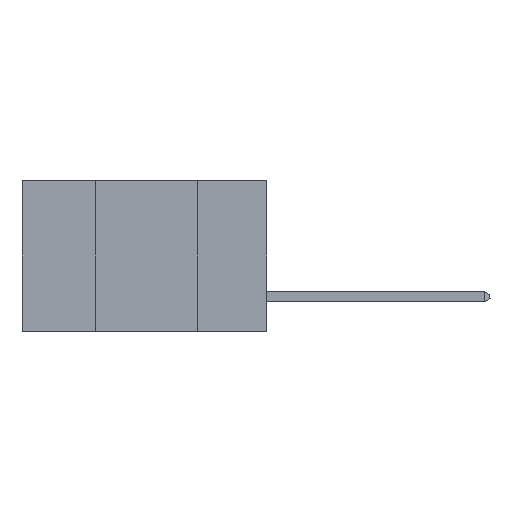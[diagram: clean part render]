
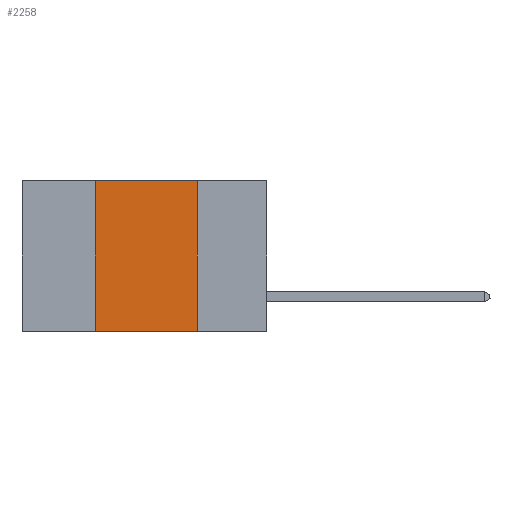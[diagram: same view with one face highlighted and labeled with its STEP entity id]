
A CAD part, left-side view. The second image highlights one B-rep face of the part: STEP entity #2258.
In plain terms, the highlighted planar face has unit normal (-1, 0, 0).
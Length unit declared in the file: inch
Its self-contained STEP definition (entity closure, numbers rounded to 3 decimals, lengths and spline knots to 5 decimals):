
#141 = ORIENTED_EDGE ( 'NONE', *, *, #20938, .F. ) ;
#144 = VERTEX_POINT ( 'NONE', #7579 ) ;
#850 = EDGE_CURVE ( 'NONE', #144, #875, #19099, .T. ) ;
#875 = VERTEX_POINT ( 'NONE', #9905 ) ;
#2085 = VECTOR ( 'NONE', #15991, 39.37008 ) ;
#2258 = ADVANCED_FACE ( 'NONE', ( #5302 ), #19737, .F. ) ;
#3033 = ORIENTED_EDGE ( 'NONE', *, *, #5304, .F. ) ;
#4265 = EDGE_LOOP ( 'NONE', ( #11182, #3033, #141, #21207 ) ) ;
#4386 = DIRECTION ( 'NONE',  ( 0., -1., 0. ) ) ;
#5198 = CARTESIAN_POINT ( 'NONE',  ( 0., 0.42, 0. ) ) ;
#5302 = FACE_OUTER_BOUND ( 'NONE', #4265, .T. ) ;
#5304 = EDGE_CURVE ( 'NONE', #12394, #144, #10483, .T. ) ;
#7237 = VECTOR ( 'NONE', #17826, 39.37008 ) ;
#7579 = CARTESIAN_POINT ( 'NONE',  ( 0., 0.17, 0. ) ) ;
#9636 = VECTOR ( 'NONE', #4386, 39.37008 ) ;
#9807 = DIRECTION ( 'NONE',  ( 1., 0., 0. ) ) ;
#9905 = CARTESIAN_POINT ( 'NONE',  ( 0., 0.17, -0.37 ) ) ;
#10110 = VECTOR ( 'NONE', #11471, 39.37008 ) ;
#10138 = CARTESIAN_POINT ( 'NONE',  ( 0., 0.6, -0.37 ) ) ;
#10392 = CARTESIAN_POINT ( 'NONE',  ( 0., 0.42, -0.37 ) ) ;
#10483 = LINE ( 'NONE', #16244, #2085 ) ;
#11182 = ORIENTED_EDGE ( 'NONE', *, *, #850, .F. ) ;
#11471 = DIRECTION ( 'NONE',  ( 0., 0., 1. ) ) ;
#11735 = CARTESIAN_POINT ( 'NONE',  ( 0., 0.17, 0. ) ) ;
#11829 = DIRECTION ( 'NONE',  ( 0., 0., -1. ) ) ;
#12394 = VERTEX_POINT ( 'NONE', #20597 ) ;
#15991 = DIRECTION ( 'NONE',  ( 0., -1., 0. ) ) ;
#16244 = CARTESIAN_POINT ( 'NONE',  ( 0., 0.6, 0. ) ) ;
#17371 = EDGE_CURVE ( 'NONE', #22527, #875, #18966, .T. ) ;
#17826 = DIRECTION ( 'NONE',  ( 0., 0., -1. ) ) ;
#18966 = LINE ( 'NONE', #10138, #9636 ) ;
#19099 = LINE ( 'NONE', #11735, #7237 ) ;
#19737 = PLANE ( 'NONE',  #23122 ) ;
#20597 = CARTESIAN_POINT ( 'NONE',  ( 0., 0.42, 0. ) ) ;
#20938 = EDGE_CURVE ( 'NONE', #22527, #12394, #23396, .T. ) ;
#21207 = ORIENTED_EDGE ( 'NONE', *, *, #17371, .T. ) ;
#22527 = VERTEX_POINT ( 'NONE', #10392 ) ;
#23122 = AXIS2_PLACEMENT_3D ( 'NONE', #23303, #9807, #11829 ) ;
#23303 = CARTESIAN_POINT ( 'NONE',  ( 0., 0.6, 0. ) ) ;
#23396 = LINE ( 'NONE', #5198, #10110 ) ;
